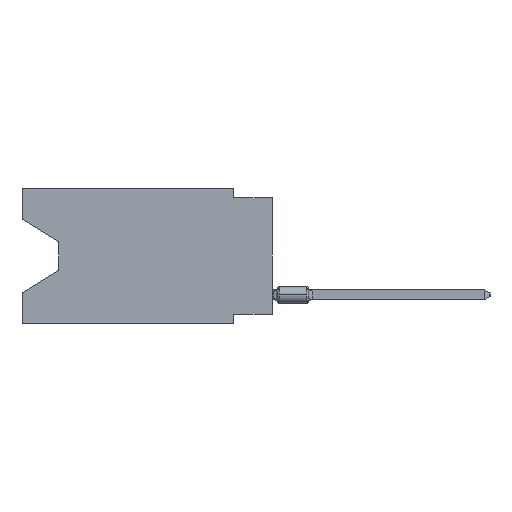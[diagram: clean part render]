
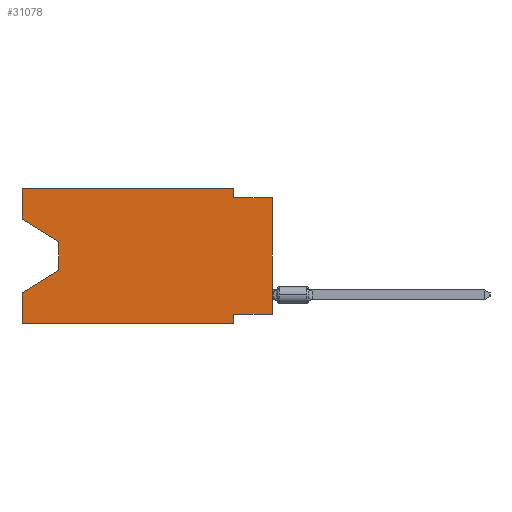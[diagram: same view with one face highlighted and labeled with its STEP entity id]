
A CAD part, left-side view. The second image highlights one B-rep face of the part: STEP entity #31078.
In plain terms, the highlighted planar face has unit normal (-1, 0, 0).
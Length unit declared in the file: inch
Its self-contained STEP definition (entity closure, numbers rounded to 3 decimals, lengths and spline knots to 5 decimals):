
#330 = VERTEX_POINT ( 'NONE', #23519 ) ;
#373 = ORIENTED_EDGE ( 'NONE', *, *, #4081, .F. ) ;
#492 = DIRECTION ( 'NONE',  ( 0., 0., 1. ) ) ;
#615 = VERTEX_POINT ( 'NONE', #23440 ) ;
#1720 = LINE ( 'NONE', #23571, #45393 ) ;
#1724 = ORIENTED_EDGE ( 'NONE', *, *, #47482, .T. ) ;
#2615 = EDGE_CURVE ( 'NONE', #615, #30859, #9362, .T. ) ;
#2721 = EDGE_CURVE ( 'NONE', #30859, #70114, #50070, .T. ) ;
#3004 = CARTESIAN_POINT ( 'NONE',  ( 0., 0.55, -0.138 ) ) ;
#3810 = CARTESIAN_POINT ( 'NONE',  ( 0., 0.645, 0. ) ) ;
#4081 = EDGE_CURVE ( 'NONE', #23629, #40890, #66733, .T. ) ;
#4313 = LINE ( 'NONE', #63670, #30424 ) ;
#4339 = DIRECTION ( 'NONE',  ( 0., 0., -1. ) ) ;
#4676 = VECTOR ( 'NONE', #6102, 39.37008 ) ;
#4921 = ORIENTED_EDGE ( 'NONE', *, *, #14554, .T. ) ;
#6102 = DIRECTION ( 'NONE',  ( 0., -1., 0. ) ) ;
#6477 = VECTOR ( 'NONE', #25509, 39.37008 ) ;
#7036 = CARTESIAN_POINT ( 'NONE',  ( 0., 0.645, 0. ) ) ;
#7317 = ORIENTED_EDGE ( 'NONE', *, *, #10142, .F. ) ;
#7773 = LINE ( 'NONE', #51053, #47905 ) ;
#8058 = ORIENTED_EDGE ( 'NONE', *, *, #33810, .F. ) ;
#8673 = LINE ( 'NONE', #20849, #6477 ) ;
#9362 = LINE ( 'NONE', #21516, #52601 ) ;
#10142 = EDGE_CURVE ( 'NONE', #40890, #615, #70298, .T. ) ;
#10557 = CARTESIAN_POINT ( 'NONE',  ( 0., 0., 0. ) ) ;
#10867 = DIRECTION ( 'NONE',  ( 0., -1., 0. ) ) ;
#14225 = FACE_OUTER_BOUND ( 'NONE', #57856, .T. ) ;
#14424 = CARTESIAN_POINT ( 'NONE',  ( 0., 0.645, -0.35 ) ) ;
#14554 = EDGE_CURVE ( 'NONE', #67051, #52128, #8673, .T. ) ;
#14703 = DIRECTION ( 'NONE',  ( 0., 1., 0. ) ) ;
#16668 = EDGE_CURVE ( 'NONE', #22917, #67051, #1720, .T. ) ;
#16852 = CARTESIAN_POINT ( 'NONE',  ( 0., 0., -0.025 ) ) ;
#17220 = VECTOR ( 'NONE', #55211, 39.37008 ) ;
#17959 = CARTESIAN_POINT ( 'NONE',  ( 0., 0., -0.325 ) ) ;
#18258 = DIRECTION ( 'NONE',  ( 0., 0., -1. ) ) ;
#18566 = DIRECTION ( 'NONE',  ( 0., 0., -1. ) ) ;
#18690 = EDGE_CURVE ( 'NONE', #54570, #52128, #7773, .T. ) ;
#20849 = CARTESIAN_POINT ( 'NONE',  ( 0., 0.55, -0.212 ) ) ;
#21413 = VECTOR ( 'NONE', #41724, 39.37008 ) ;
#21516 = CARTESIAN_POINT ( 'NONE',  ( 0., 0.1, 0. ) ) ;
#21820 = EDGE_CURVE ( 'NONE', #23629, #22917, #54862, .T. ) ;
#22917 = VERTEX_POINT ( 'NONE', #3004 ) ;
#23234 = AXIS2_PLACEMENT_3D ( 'NONE', #33974, #36016, #18258 ) ;
#23440 = CARTESIAN_POINT ( 'NONE',  ( 0., 0.1, 0. ) ) ;
#23519 = CARTESIAN_POINT ( 'NONE',  ( 0., 0.1, -0.325 ) ) ;
#23571 = CARTESIAN_POINT ( 'NONE',  ( 0., 0.55, -0.138 ) ) ;
#23629 = VERTEX_POINT ( 'NONE', #62147 ) ;
#25509 = DIRECTION ( 'NONE',  ( 0., 0.855, -0.519 ) ) ;
#25919 = VERTEX_POINT ( 'NONE', #31923 ) ;
#28952 = VECTOR ( 'NONE', #10867, 39.37008 ) ;
#30424 = VECTOR ( 'NONE', #14703, 39.37008 ) ;
#30859 = VERTEX_POINT ( 'NONE', #59064 ) ;
#31078 = ADVANCED_FACE ( 'NONE', ( #14225 ), #50441, .F. ) ;
#31546 = VECTOR ( 'NONE', #18566, 39.37008 ) ;
#31923 = CARTESIAN_POINT ( 'NONE',  ( 0., 0.1, -0.35 ) ) ;
#33810 = EDGE_CURVE ( 'NONE', #330, #25919, #55725, .T. ) ;
#33974 = CARTESIAN_POINT ( 'NONE',  ( 0., 0.645, 0. ) ) ;
#34608 = DIRECTION ( 'NONE',  ( 0., 0., 1. ) ) ;
#34927 = ORIENTED_EDGE ( 'NONE', *, *, #2721, .F. ) ;
#35325 = VECTOR ( 'NONE', #492, 39.37008 ) ;
#36016 = DIRECTION ( 'NONE',  ( 1., 0., 0. ) ) ;
#39284 = CARTESIAN_POINT ( 'NONE',  ( 0., 0.1, -0.35 ) ) ;
#39562 = CARTESIAN_POINT ( 'NONE',  ( 0., 0.645, -0.26975 ) ) ;
#39704 = CARTESIAN_POINT ( 'NONE',  ( 0., 0.55, -0.212 ) ) ;
#40890 = VERTEX_POINT ( 'NONE', #42693 ) ;
#41724 = DIRECTION ( 'NONE',  ( 0., -1., 0. ) ) ;
#42693 = CARTESIAN_POINT ( 'NONE',  ( 0., 0.645, 0. ) ) ;
#45384 = DIRECTION ( 'NONE',  ( 0., 0., -1. ) ) ;
#45393 = VECTOR ( 'NONE', #45384, 39.37008 ) ;
#47482 = EDGE_CURVE ( 'NONE', #54570, #25919, #65219, .T. ) ;
#47828 = ORIENTED_EDGE ( 'NONE', *, *, #55930, .T. ) ;
#47905 = VECTOR ( 'NONE', #34608, 39.37008 ) ;
#49846 = CARTESIAN_POINT ( 'NONE',  ( 0., 0.645, -0.08025 ) ) ;
#50045 = CARTESIAN_POINT ( 'NONE',  ( 0., 0., -0.025 ) ) ;
#50070 = LINE ( 'NONE', #16852, #4676 ) ;
#50313 = DIRECTION ( 'NONE',  ( 0., 0., 1. ) ) ;
#50441 = PLANE ( 'NONE',  #23234 ) ;
#51053 = CARTESIAN_POINT ( 'NONE',  ( 0., 0.645, 0. ) ) ;
#52128 = VERTEX_POINT ( 'NONE', #39562 ) ;
#52601 = VECTOR ( 'NONE', #4339, 39.37008 ) ;
#52807 = EDGE_CURVE ( 'NONE', #58075, #330, #4313, .T. ) ;
#54570 = VERTEX_POINT ( 'NONE', #14424 ) ;
#54838 = CARTESIAN_POINT ( 'NONE',  ( 0., 0.645, -0.35 ) ) ;
#54862 = LINE ( 'NONE', #49846, #17220 ) ;
#55211 = DIRECTION ( 'NONE',  ( 0., -0.855, -0.519 ) ) ;
#55725 = LINE ( 'NONE', #39284, #31546 ) ;
#55930 = EDGE_CURVE ( 'NONE', #58075, #70114, #60587, .T. ) ;
#57856 = EDGE_LOOP ( 'NONE', ( #61810, #69585, #4921, #59649, #1724, #8058, #59222, #47828, #34927, #69679, #7317, #373 ) ) ;
#58075 = VERTEX_POINT ( 'NONE', #17959 ) ;
#59064 = CARTESIAN_POINT ( 'NONE',  ( 0., 0.1, -0.025 ) ) ;
#59222 = ORIENTED_EDGE ( 'NONE', *, *, #52807, .F. ) ;
#59352 = VECTOR ( 'NONE', #50313, 39.37008 ) ;
#59649 = ORIENTED_EDGE ( 'NONE', *, *, #18690, .F. ) ;
#60587 = LINE ( 'NONE', #10557, #35325 ) ;
#61810 = ORIENTED_EDGE ( 'NONE', *, *, #21820, .T. ) ;
#62147 = CARTESIAN_POINT ( 'NONE',  ( 0., 0.645, -0.08025 ) ) ;
#63670 = CARTESIAN_POINT ( 'NONE',  ( 0., 0., -0.325 ) ) ;
#65219 = LINE ( 'NONE', #54838, #28952 ) ;
#66733 = LINE ( 'NONE', #7036, #59352 ) ;
#67051 = VERTEX_POINT ( 'NONE', #39704 ) ;
#69585 = ORIENTED_EDGE ( 'NONE', *, *, #16668, .T. ) ;
#69679 = ORIENTED_EDGE ( 'NONE', *, *, #2615, .F. ) ;
#70114 = VERTEX_POINT ( 'NONE', #50045 ) ;
#70298 = LINE ( 'NONE', #3810, #21413 ) ;
